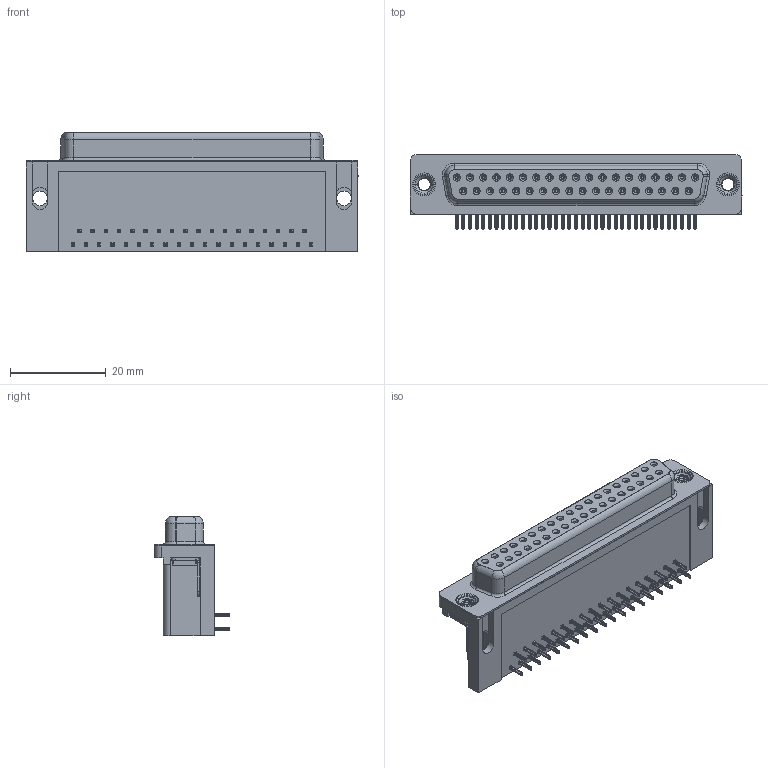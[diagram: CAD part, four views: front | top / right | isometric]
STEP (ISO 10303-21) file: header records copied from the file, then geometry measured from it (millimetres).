
FILE_DESCRIPTION (( 'STEP AP203' ), '1' );
FILE_NAME ('626-037-262-515.STEP', '2018-11-07T05:05:58', ( '' ), ( '' ), 'SwSTEP 2.0', 'SolidWorks 2016', '' );
FILE_SCHEMA (( 'CONFIG_CONTROL_DESIGN' ));
Length unit declared in the file: millimetre
Products named in the file (7): 626 Thru Hole Board Mount; 626 M3 Threaded Rivet; 626-037-262-515; 626 Housing_37 Socket; 626 Shell_37 Socket; 626 Contact Bottom; 626 Contact Top
Assembly tree (43 placements, depth 2):
  626-037-262-515
    626 Housing_37 Socket
    626 Shell_37 Socket
    626 Contact Bottom  x18
    626 Contact Top  x19
    626 Thru Hole Board Mount  x2
    626 M3 Threaded Rivet  x2
Bounding box: 69.4 x 15.73 x 24.96 mm (x, y, z)
Volume: 14702.7 mm3; surface area: 15327.4 mm2
Topology: 43 solids, 43 shells, 5560 faces, 14594 edges, 9146 vertices
Faces by surface type: plane 2502, cylinder 1302, bspline 1266, cone 452, torus 38
Entity records: 35947 total; most frequent: CARTESIAN_POINT 10249, ORIENTED_EDGE 5030, DIRECTION 4734, EDGE_CURVE 2515, VECTOR 1702, LINE 1702, VERTEX_POINT 1609, AXIS2_PLACEMENT_3D 1516
